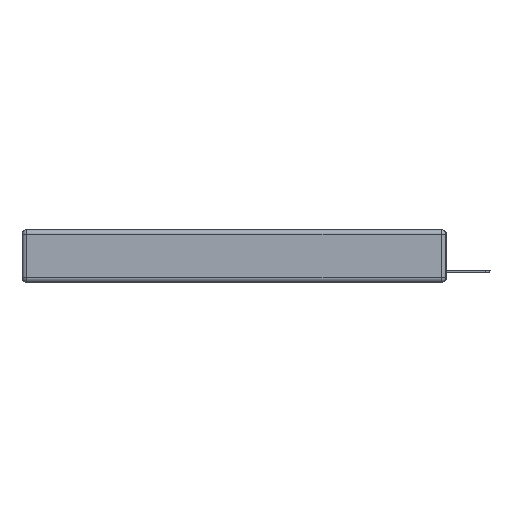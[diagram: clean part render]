
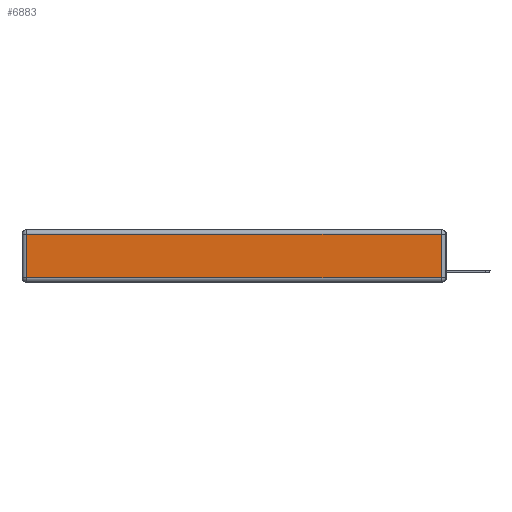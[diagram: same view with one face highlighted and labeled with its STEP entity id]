
A CAD part, left-side view. The second image highlights one B-rep face of the part: STEP entity #6883.
In plain terms, the highlighted planar face has unit normal (-1, 0, 0).
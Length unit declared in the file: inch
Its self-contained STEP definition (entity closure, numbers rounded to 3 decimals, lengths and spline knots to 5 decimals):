
#3 = LINE ( 'NONE', #17865, #4276 ) ;
#1396 = VECTOR ( 'NONE', #6141, 39.37008 ) ;
#1642 = VERTEX_POINT ( 'NONE', #9069 ) ;
#1662 = ORIENTED_EDGE ( 'NONE', *, *, #15085, .T. ) ;
#2247 = AXIS2_PLACEMENT_3D ( 'NONE', #22205, #8138, #8060 ) ;
#2579 = VERTEX_POINT ( 'NONE', #7619 ) ;
#2731 = CARTESIAN_POINT ( 'NONE',  ( 0., 2.72, -0.313 ) ) ;
#3403 = LINE ( 'NONE', #8557, #10694 ) ;
#4276 = VECTOR ( 'NONE', #6982, 39.37008 ) ;
#5021 = FACE_OUTER_BOUND ( 'NONE', #22298, .T. ) ;
#5672 = DIRECTION ( 'NONE',  ( 0., -1., 0. ) ) ;
#5713 = EDGE_CURVE ( 'NONE', #12848, #20492, #12359, .T. ) ;
#6141 = DIRECTION ( 'NONE',  ( 0., 0., -1. ) ) ;
#6883 = ADVANCED_FACE ( 'NONE', ( #5021 ), #18728, .T. ) ;
#6982 = DIRECTION ( 'NONE',  ( 0., 0., 1. ) ) ;
#7619 = CARTESIAN_POINT ( 'NONE',  ( 0., 0.03, -0.03 ) ) ;
#8060 = DIRECTION ( 'NONE',  ( 0., 0., 1. ) ) ;
#8138 = DIRECTION ( 'NONE',  ( -1., 0., 0. ) ) ;
#8557 = CARTESIAN_POINT ( 'NONE',  ( 0., 2.75, -0.03 ) ) ;
#9069 = CARTESIAN_POINT ( 'NONE',  ( 0., 0.03, -0.313 ) ) ;
#9617 = ORIENTED_EDGE ( 'NONE', *, *, #5713, .T. ) ;
#9681 = CARTESIAN_POINT ( 'NONE',  ( 0., 2.72, -0.343 ) ) ;
#10694 = VECTOR ( 'NONE', #22859, 39.37008 ) ;
#12359 = LINE ( 'NONE', #9681, #1396 ) ;
#12842 = EDGE_CURVE ( 'NONE', #1642, #2579, #3, .T. ) ;
#12848 = VERTEX_POINT ( 'NONE', #14171 ) ;
#14171 = CARTESIAN_POINT ( 'NONE',  ( 0., 2.72, -0.03 ) ) ;
#14762 = CARTESIAN_POINT ( 'NONE',  ( 0., 0., -0.313 ) ) ;
#15085 = EDGE_CURVE ( 'NONE', #20492, #1642, #23262, .T. ) ;
#15665 = ORIENTED_EDGE ( 'NONE', *, *, #20566, .T. ) ;
#17865 = CARTESIAN_POINT ( 'NONE',  ( 0., 0.03, -0.343 ) ) ;
#18450 = VECTOR ( 'NONE', #5672, 39.37008 ) ;
#18728 = PLANE ( 'NONE',  #2247 ) ;
#20492 = VERTEX_POINT ( 'NONE', #2731 ) ;
#20566 = EDGE_CURVE ( 'NONE', #2579, #12848, #3403, .T. ) ;
#22205 = CARTESIAN_POINT ( 'NONE',  ( 0., 0., -0.343 ) ) ;
#22298 = EDGE_LOOP ( 'NONE', ( #1662, #23125, #15665, #9617 ) ) ;
#22859 = DIRECTION ( 'NONE',  ( 0., 1., 0. ) ) ;
#23125 = ORIENTED_EDGE ( 'NONE', *, *, #12842, .T. ) ;
#23262 = LINE ( 'NONE', #14762, #18450 ) ;
